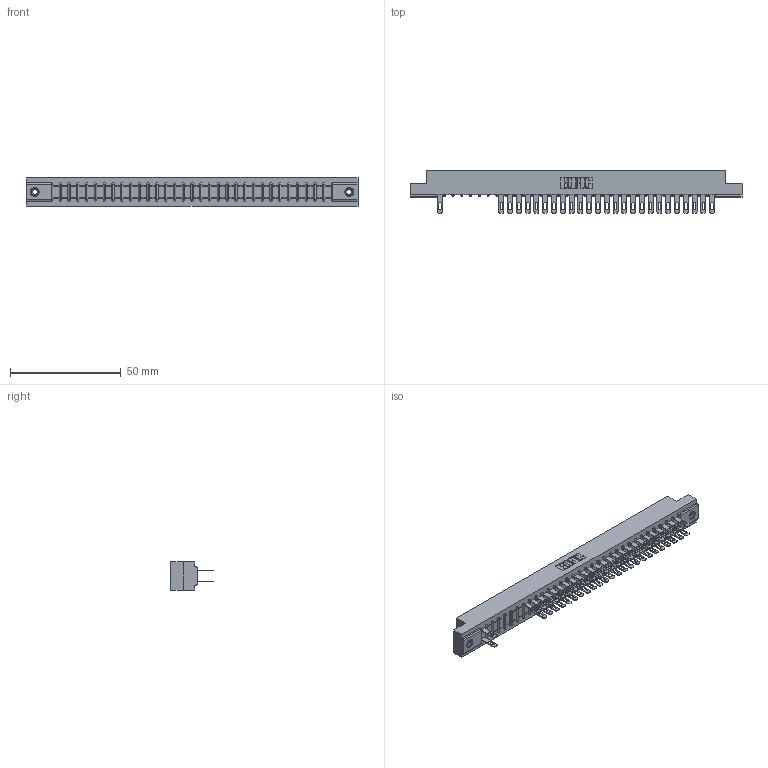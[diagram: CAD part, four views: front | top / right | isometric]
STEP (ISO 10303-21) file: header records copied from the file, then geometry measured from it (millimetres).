
FILE_DESCRIPTION (( 'STEP AP203' ), '1' );
FILE_NAME ('307-064-500-208.STEP', '2018-08-06T09:51:43', ( '' ), ( '' ), 'SwSTEP 2.0', 'SolidWorks 2016', '' );
FILE_SCHEMA (( 'CONFIG_CONTROL_DESIGN' ));
Length unit declared in the file: inch
Products named in the file (4): 345-250-001_345-250-003-102; 307-064-500-208; 307 Part_.156 Dia Mounting Holes; 307-290-001_500
Assembly tree (54 placements, depth 2):
  307-064-500-208
    307 Part_.156 Dia Mounting Holes
    307-290-001_500  x51
    345-250-001_345-250-003-102  x2
Bounding box: 149.81 x 19.18 x 12.7 mm (x, y, z)
Volume: 15830.9 mm3; surface area: 18895.1 mm2
Topology: 54 solids, 54 shells, 2687 faces, 7505 edges, 4838 vertices
Faces by surface type: plane 1710, cylinder 895, sphere 66, cone 12, torus 4
Entity records: 30433 total; most frequent: CARTESIAN_POINT 5018, ORIENTED_EDGE 4978, DIRECTION 4917, EDGE_CURVE 2489, LINE 1903, VECTOR 1903, VERTEX_POINT 1608, AXIS2_PLACEMENT_3D 1507
